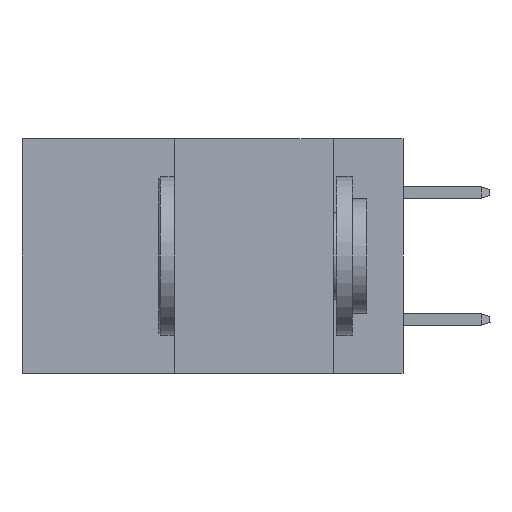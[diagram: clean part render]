
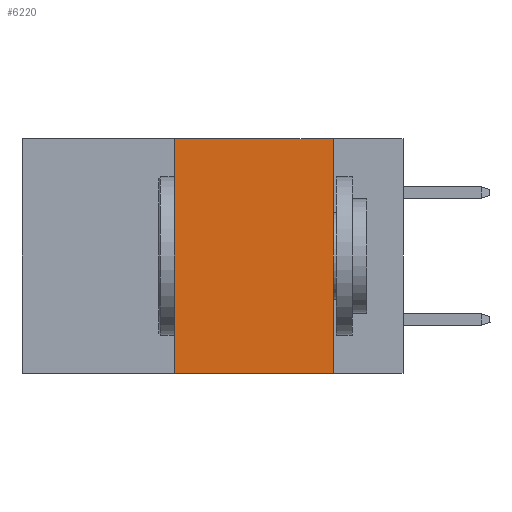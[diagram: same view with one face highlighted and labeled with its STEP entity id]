
A CAD part, left-side view. The second image highlights one B-rep face of the part: STEP entity #6220.
In plain terms, the highlighted planar face has unit normal (-1, 0, 0).
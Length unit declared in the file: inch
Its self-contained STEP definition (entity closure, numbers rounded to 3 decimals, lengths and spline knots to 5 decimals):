
#999 = DIRECTION ( 'NONE',  ( 0., 0., 1. ) ) ;
#2106 = CARTESIAN_POINT ( 'NONE',  ( 0., 0.11, -0.37 ) ) ;
#2623 = VERTEX_POINT ( 'NONE', #16300 ) ;
#4240 = EDGE_CURVE ( 'NONE', #21907, #14849, #27556, .T. ) ;
#4453 = DIRECTION ( 'NONE',  ( 0., 0., -1. ) ) ;
#6220 = ADVANCED_FACE ( 'NONE', ( #28558 ), #28375, .F. ) ;
#6714 = EDGE_CURVE ( 'NONE', #21907, #34351, #10167, .T. ) ;
#7637 = CARTESIAN_POINT ( 'NONE',  ( 0., 0.6, 0. ) ) ;
#9196 = CARTESIAN_POINT ( 'NONE',  ( 0., 0.36, 0. ) ) ;
#9662 = VECTOR ( 'NONE', #30771, 39.37008 ) ;
#9907 = DIRECTION ( 'NONE',  ( 0., -1., 0. ) ) ;
#10167 = LINE ( 'NONE', #20467, #9662 ) ;
#12002 = EDGE_CURVE ( 'NONE', #14849, #2623, #15508, .T. ) ;
#12309 = DIRECTION ( 'NONE',  ( 1., 0., 0. ) ) ;
#12659 = DIRECTION ( 'NONE',  ( 0., 0., -1. ) ) ;
#12669 = ORIENTED_EDGE ( 'NONE', *, *, #23655, .F. ) ;
#14830 = ORIENTED_EDGE ( 'NONE', *, *, #4240, .F. ) ;
#14849 = VERTEX_POINT ( 'NONE', #30060 ) ;
#15277 = CARTESIAN_POINT ( 'NONE',  ( 0., 0.6, 0. ) ) ;
#15508 = LINE ( 'NONE', #7637, #22632 ) ;
#16300 = CARTESIAN_POINT ( 'NONE',  ( 0., 0.11, 0. ) ) ;
#20467 = CARTESIAN_POINT ( 'NONE',  ( 0., 0.6, -0.37 ) ) ;
#21148 = VECTOR ( 'NONE', #999, 39.37008 ) ;
#21868 = ORIENTED_EDGE ( 'NONE', *, *, #6714, .T. ) ;
#21907 = VERTEX_POINT ( 'NONE', #23315 ) ;
#22632 = VECTOR ( 'NONE', #9907, 39.37008 ) ;
#23315 = CARTESIAN_POINT ( 'NONE',  ( 0., 0.36, -0.37 ) ) ;
#23655 = EDGE_CURVE ( 'NONE', #2623, #34351, #30823, .T. ) ;
#25686 = AXIS2_PLACEMENT_3D ( 'NONE', #15277, #12309, #12659 ) ;
#25807 = VECTOR ( 'NONE', #4453, 39.37008 ) ;
#27556 = LINE ( 'NONE', #9196, #21148 ) ;
#28231 = ORIENTED_EDGE ( 'NONE', *, *, #12002, .F. ) ;
#28375 = PLANE ( 'NONE',  #25686 ) ;
#28558 = FACE_OUTER_BOUND ( 'NONE', #30555, .T. ) ;
#30060 = CARTESIAN_POINT ( 'NONE',  ( 0., 0.36, 0. ) ) ;
#30555 = EDGE_LOOP ( 'NONE', ( #12669, #28231, #14830, #21868 ) ) ;
#30771 = DIRECTION ( 'NONE',  ( 0., -1., 0. ) ) ;
#30823 = LINE ( 'NONE', #31831, #25807 ) ;
#31831 = CARTESIAN_POINT ( 'NONE',  ( 0., 0.11, 0. ) ) ;
#34351 = VERTEX_POINT ( 'NONE', #2106 ) ;
